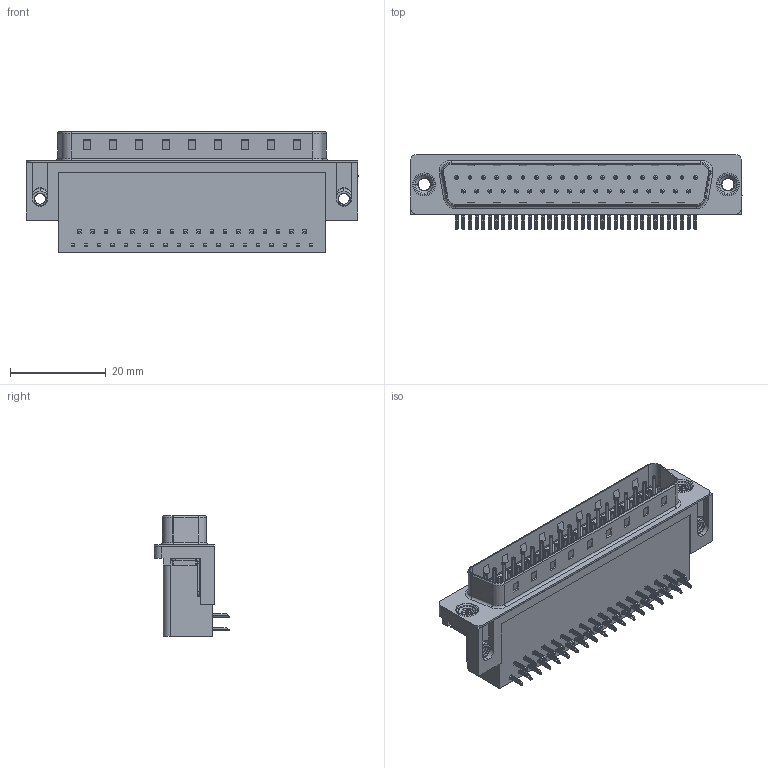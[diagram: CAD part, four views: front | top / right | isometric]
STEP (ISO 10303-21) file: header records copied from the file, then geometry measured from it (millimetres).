
FILE_DESCRIPTION (( 'STEP AP203' ), '1' );
FILE_NAME ('625-037-362-055.STEP', '2018-11-06T05:43:45', ( '' ), ( '' ), 'SwSTEP 2.0', 'SolidWorks 2016', '' );
FILE_SCHEMA (( 'CONFIG_CONTROL_DESIGN' ));
Length unit declared in the file: millimetre
Products named in the file (7): 625 Contact Top; 625 M3 Threaded Rivet; 625 4-40 Threaded Board Mount; 625-037-362-055; 625 Housing_37 Socket; 625 Shell_37 Socket; 625 Contact Bottom
Assembly tree (43 placements, depth 2):
  625-037-362-055
    625 Housing_37 Socket
    625 Shell_37 Socket
    625 Contact Bottom  x18
    625 Contact Top  x19
    625 4-40 Threaded Board Mount  x2
    625 M3 Threaded Rivet  x2
Bounding box: 69.4 x 15.73 x 25.16 mm (x, y, z)
Volume: 12606.3 mm3; surface area: 11836.9 mm2
Topology: 43 solids, 43 shells, 3233 faces, 7997 edges, 4933 vertices
Faces by surface type: plane 2015, cylinder 933, torus 265, bspline 12, cone 8
Entity records: 28414 total; most frequent: CARTESIAN_POINT 7039, DIRECTION 4121, ORIENTED_EDGE 3998, EDGE_CURVE 1999, VECTOR 1421, LINE 1421, AXIS2_PLACEMENT_3D 1350, VERTEX_POINT 1288
